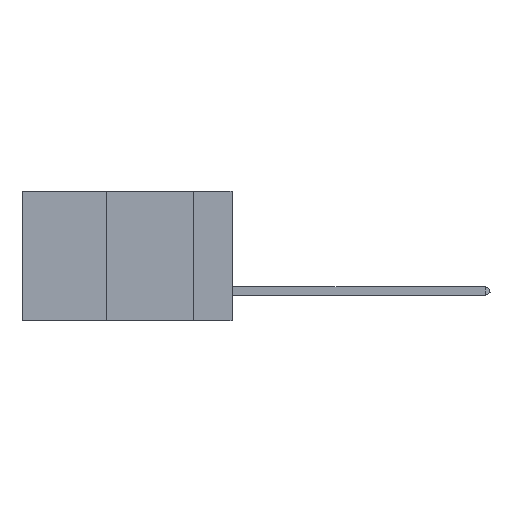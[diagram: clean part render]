
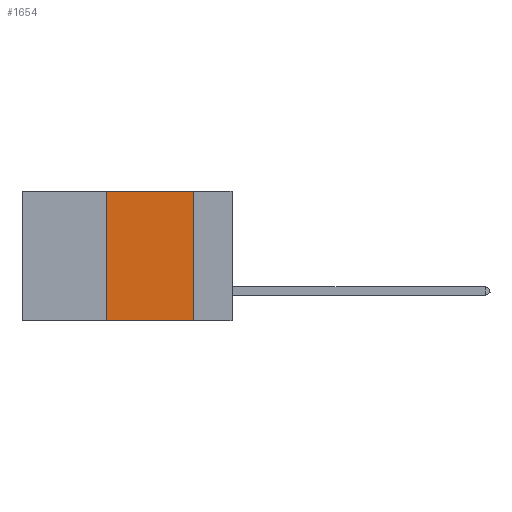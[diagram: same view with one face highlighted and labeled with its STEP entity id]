
A CAD part, left-side view. The second image highlights one B-rep face of the part: STEP entity #1654.
In plain terms, the highlighted planar face has unit normal (-1, 0, 0).
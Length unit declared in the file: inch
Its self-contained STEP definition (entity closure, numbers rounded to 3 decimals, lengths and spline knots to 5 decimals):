
#124 = LINE ( 'NONE', #11886, #7318 ) ;
#948 = VERTEX_POINT ( 'NONE', #5075 ) ;
#1341 = CARTESIAN_POINT ( 'NONE',  ( 0., 0.11, -0.37 ) ) ;
#1627 = DIRECTION ( 'NONE',  ( 0., 0., 1. ) ) ;
#1654 = ADVANCED_FACE ( 'NONE', ( #16235 ), #3842, .F. ) ;
#3456 = ORIENTED_EDGE ( 'NONE', *, *, #7884, .F. ) ;
#3842 = PLANE ( 'NONE',  #12884 ) ;
#4317 = VERTEX_POINT ( 'NONE', #11451 ) ;
#5075 = CARTESIAN_POINT ( 'NONE',  ( 0., 0.36, 0. ) ) ;
#5385 = CARTESIAN_POINT ( 'NONE',  ( 0., 0.6, 0. ) ) ;
#5677 = EDGE_CURVE ( 'NONE', #948, #5684, #7385, .T. ) ;
#5684 = VERTEX_POINT ( 'NONE', #18684 ) ;
#5888 = DIRECTION ( 'NONE',  ( 0., 0., -1. ) ) ;
#6818 = CARTESIAN_POINT ( 'NONE',  ( 0., 0.6, 0. ) ) ;
#6853 = DIRECTION ( 'NONE',  ( 0., -1., 0. ) ) ;
#7022 = LINE ( 'NONE', #16998, #13742 ) ;
#7318 = VECTOR ( 'NONE', #1627, 39.37008 ) ;
#7385 = LINE ( 'NONE', #5385, #9232 ) ;
#7884 = EDGE_CURVE ( 'NONE', #5684, #9913, #9372, .T. ) ;
#8632 = EDGE_CURVE ( 'NONE', #4317, #9913, #7022, .T. ) ;
#8896 = VECTOR ( 'NONE', #5888, 39.37008 ) ;
#9232 = VECTOR ( 'NONE', #6853, 39.37008 ) ;
#9372 = LINE ( 'NONE', #15144, #8896 ) ;
#9913 = VERTEX_POINT ( 'NONE', #1341 ) ;
#11450 = EDGE_LOOP ( 'NONE', ( #3456, #13658, #18486, #13545 ) ) ;
#11451 = CARTESIAN_POINT ( 'NONE',  ( 0., 0.36, -0.37 ) ) ;
#11886 = CARTESIAN_POINT ( 'NONE',  ( 0., 0.36, 0. ) ) ;
#12475 = DIRECTION ( 'NONE',  ( 0., -1., 0. ) ) ;
#12884 = AXIS2_PLACEMENT_3D ( 'NONE', #6818, #18464, #17180 ) ;
#13545 = ORIENTED_EDGE ( 'NONE', *, *, #8632, .T. ) ;
#13658 = ORIENTED_EDGE ( 'NONE', *, *, #5677, .F. ) ;
#13742 = VECTOR ( 'NONE', #12475, 39.37008 ) ;
#15144 = CARTESIAN_POINT ( 'NONE',  ( 0., 0.11, 0. ) ) ;
#16235 = FACE_OUTER_BOUND ( 'NONE', #11450, .T. ) ;
#16968 = EDGE_CURVE ( 'NONE', #4317, #948, #124, .T. ) ;
#16998 = CARTESIAN_POINT ( 'NONE',  ( 0., 0.6, -0.37 ) ) ;
#17180 = DIRECTION ( 'NONE',  ( 0., 0., -1. ) ) ;
#18464 = DIRECTION ( 'NONE',  ( 1., 0., 0. ) ) ;
#18486 = ORIENTED_EDGE ( 'NONE', *, *, #16968, .F. ) ;
#18684 = CARTESIAN_POINT ( 'NONE',  ( 0., 0.11, 0. ) ) ;
